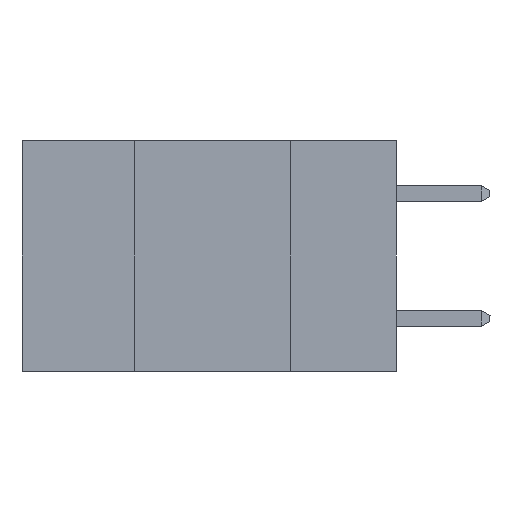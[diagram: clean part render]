
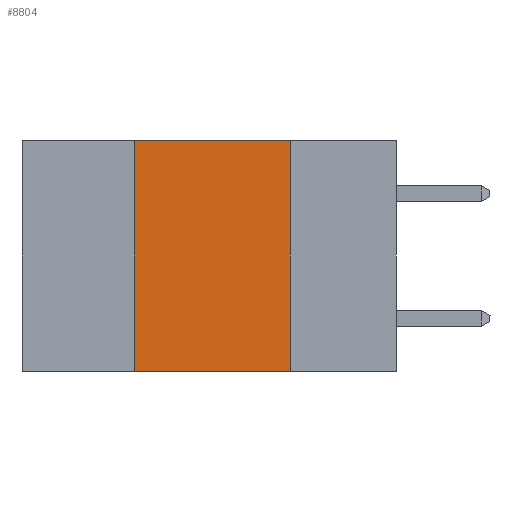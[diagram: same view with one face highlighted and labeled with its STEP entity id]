
A CAD part, left-side view. The second image highlights one B-rep face of the part: STEP entity #8804.
In plain terms, the highlighted planar face has unit normal (-1, 0, 0).
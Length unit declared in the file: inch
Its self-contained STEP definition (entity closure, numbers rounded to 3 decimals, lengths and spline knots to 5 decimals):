
#154 = VERTEX_POINT ( 'NONE', #10805 ) ;
#225 = VECTOR ( 'NONE', #5256, 39.37008 ) ;
#550 = VERTEX_POINT ( 'NONE', #5426 ) ;
#760 = CARTESIAN_POINT ( 'NONE',  ( 0., 0.42, 0. ) ) ;
#830 = CARTESIAN_POINT ( 'NONE',  ( 0., 0.6, 0. ) ) ;
#1669 = ORIENTED_EDGE ( 'NONE', *, *, #23517, .F. ) ;
#4903 = VERTEX_POINT ( 'NONE', #27819 ) ;
#5256 = DIRECTION ( 'NONE',  ( 0., -1., 0. ) ) ;
#5426 = CARTESIAN_POINT ( 'NONE',  ( 0., 0.42, -0.37 ) ) ;
#8028 = LINE ( 'NONE', #760, #8711 ) ;
#8175 = EDGE_LOOP ( 'NONE', ( #28554, #8897, #1669, #19419 ) ) ;
#8711 = VECTOR ( 'NONE', #16417, 39.37008 ) ;
#8804 = ADVANCED_FACE ( 'NONE', ( #16577 ), #20817, .F. ) ;
#8857 = CARTESIAN_POINT ( 'NONE',  ( 0., 0.17, 0. ) ) ;
#8897 = ORIENTED_EDGE ( 'NONE', *, *, #23174, .F. ) ;
#10805 = CARTESIAN_POINT ( 'NONE',  ( 0., 0.42, 0. ) ) ;
#11231 = DIRECTION ( 'NONE',  ( 0., 0., -1. ) ) ;
#11952 = DIRECTION ( 'NONE',  ( 0., 0., -1. ) ) ;
#12163 = CARTESIAN_POINT ( 'NONE',  ( 0., 0.6, 0. ) ) ;
#13589 = CARTESIAN_POINT ( 'NONE',  ( 0., 0.17, 0. ) ) ;
#15875 = LINE ( 'NONE', #25459, #225 ) ;
#16417 = DIRECTION ( 'NONE',  ( 0., 0., 1. ) ) ;
#16577 = FACE_OUTER_BOUND ( 'NONE', #8175, .T. ) ;
#17129 = VECTOR ( 'NONE', #11231, 39.37008 ) ;
#17962 = EDGE_CURVE ( 'NONE', #550, #4903, #15875, .T. ) ;
#18871 = DIRECTION ( 'NONE',  ( 1., 0., 0. ) ) ;
#19419 = ORIENTED_EDGE ( 'NONE', *, *, #17962, .T. ) ;
#20287 = LINE ( 'NONE', #13589, #17129 ) ;
#20817 = PLANE ( 'NONE',  #23384 ) ;
#20985 = DIRECTION ( 'NONE',  ( 0., -1., 0. ) ) ;
#21507 = EDGE_CURVE ( 'NONE', #23412, #4903, #20287, .T. ) ;
#22000 = VECTOR ( 'NONE', #20985, 39.37008 ) ;
#23174 = EDGE_CURVE ( 'NONE', #154, #23412, #24438, .T. ) ;
#23384 = AXIS2_PLACEMENT_3D ( 'NONE', #12163, #18871, #11952 ) ;
#23412 = VERTEX_POINT ( 'NONE', #8857 ) ;
#23517 = EDGE_CURVE ( 'NONE', #550, #154, #8028, .T. ) ;
#24438 = LINE ( 'NONE', #830, #22000 ) ;
#25459 = CARTESIAN_POINT ( 'NONE',  ( 0., 0.6, -0.37 ) ) ;
#27819 = CARTESIAN_POINT ( 'NONE',  ( 0., 0.17, -0.37 ) ) ;
#28554 = ORIENTED_EDGE ( 'NONE', *, *, #21507, .F. ) ;
